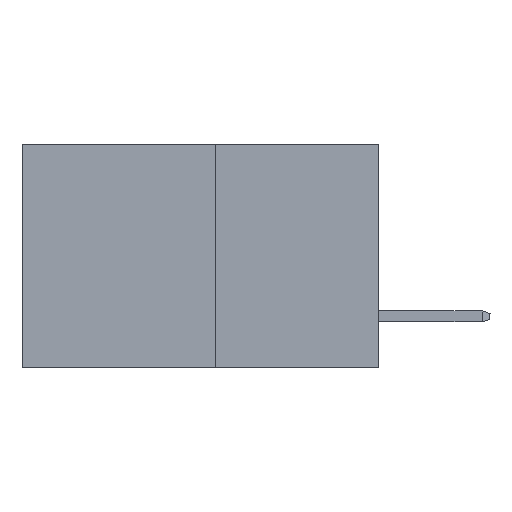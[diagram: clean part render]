
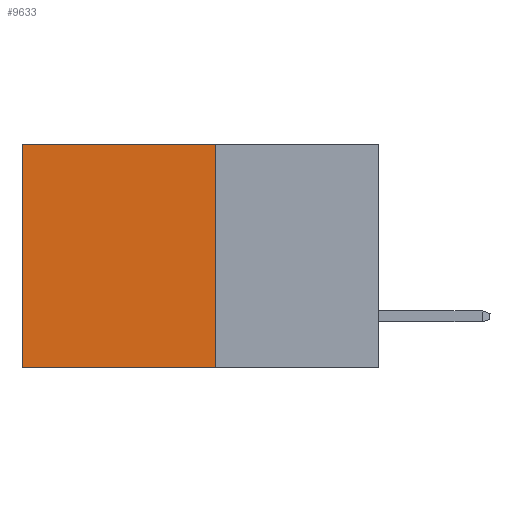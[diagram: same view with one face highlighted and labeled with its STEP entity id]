
A CAD part, left-side view. The second image highlights one B-rep face of the part: STEP entity #9633.
In plain terms, the highlighted planar face has unit normal (-1, 0, 0).
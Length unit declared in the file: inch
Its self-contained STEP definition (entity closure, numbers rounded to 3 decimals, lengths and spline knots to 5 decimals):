
#423 = VERTEX_POINT ( 'NONE', #1305 ) ;
#537 = EDGE_CURVE ( 'NONE', #423, #2567, #9952, .T. ) ;
#652 = ORIENTED_EDGE ( 'NONE', *, *, #537, .T. ) ;
#692 = CARTESIAN_POINT ( 'NONE',  ( 0.277, 0.59, -0.37 ) ) ;
#699 = LINE ( 'NONE', #700, #8296 ) ;
#700 = CARTESIAN_POINT ( 'NONE',  ( 0.277, 0.27, -0.37 ) ) ;
#752 = DIRECTION ( 'NONE',  ( 0., 0., -1. ) ) ;
#1305 = CARTESIAN_POINT ( 'NONE',  ( 0.277, 0.59, 0. ) ) ;
#2059 = DIRECTION ( 'NONE',  ( 0., 0., -1. ) ) ;
#2567 = VERTEX_POINT ( 'NONE', #9706 ) ;
#4563 = FACE_OUTER_BOUND ( 'NONE', #8595, .T. ) ;
#5175 = LINE ( 'NONE', #11283, #10309 ) ;
#5363 = EDGE_CURVE ( 'NONE', #12865, #5427, #5175, .T. ) ;
#5427 = VERTEX_POINT ( 'NONE', #10602 ) ;
#5430 = EDGE_CURVE ( 'NONE', #12865, #423, #10009, .T. ) ;
#6106 = ORIENTED_EDGE ( 'NONE', *, *, #10626, .F. ) ;
#6618 = VECTOR ( 'NONE', #10660, 39.37008 ) ;
#7205 = PLANE ( 'NONE',  #10558 ) ;
#8258 = DIRECTION ( 'NONE',  ( 1., 0., 0. ) ) ;
#8296 = VECTOR ( 'NONE', #8973, 39.37008 ) ;
#8595 = EDGE_LOOP ( 'NONE', ( #652, #6106, #8894, #9220 ) ) ;
#8894 = ORIENTED_EDGE ( 'NONE', *, *, #5363, .F. ) ;
#8973 = DIRECTION ( 'NONE',  ( 0., 1., 0. ) ) ;
#9220 = ORIENTED_EDGE ( 'NONE', *, *, #5430, .T. ) ;
#9633 = ADVANCED_FACE ( 'NONE', ( #4563 ), #7205, .F. ) ;
#9706 = CARTESIAN_POINT ( 'NONE',  ( 0.277, 0.59, -0.37 ) ) ;
#9952 = LINE ( 'NONE', #692, #12555 ) ;
#10009 = LINE ( 'NONE', #10506, #6618 ) ;
#10309 = VECTOR ( 'NONE', #11735, 39.37008 ) ;
#10506 = CARTESIAN_POINT ( 'NONE',  ( 0.277, 0.27, 0. ) ) ;
#10558 = AXIS2_PLACEMENT_3D ( 'NONE', #13184, #8258, #2059 ) ;
#10602 = CARTESIAN_POINT ( 'NONE',  ( 0.277, 0.27, -0.37 ) ) ;
#10626 = EDGE_CURVE ( 'NONE', #5427, #2567, #699, .T. ) ;
#10660 = DIRECTION ( 'NONE',  ( 0., 1., 0. ) ) ;
#11097 = CARTESIAN_POINT ( 'NONE',  ( 0.277, 0.27, 0. ) ) ;
#11283 = CARTESIAN_POINT ( 'NONE',  ( 0.277, 0.27, -0.37 ) ) ;
#11735 = DIRECTION ( 'NONE',  ( 0., 0., -1. ) ) ;
#12555 = VECTOR ( 'NONE', #752, 39.37008 ) ;
#12865 = VERTEX_POINT ( 'NONE', #11097 ) ;
#13184 = CARTESIAN_POINT ( 'NONE',  ( 0.277, 0.27, -0.37 ) ) ;
